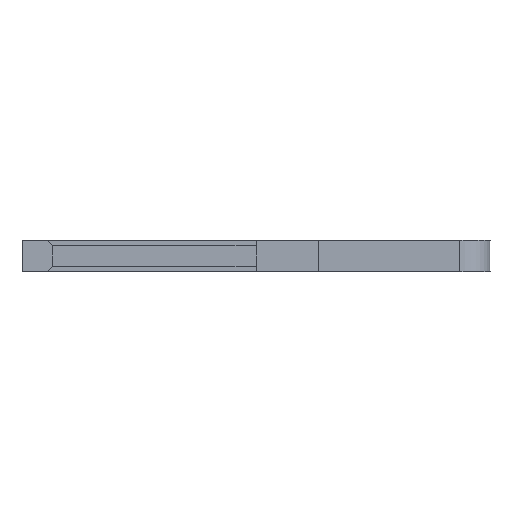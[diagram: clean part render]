
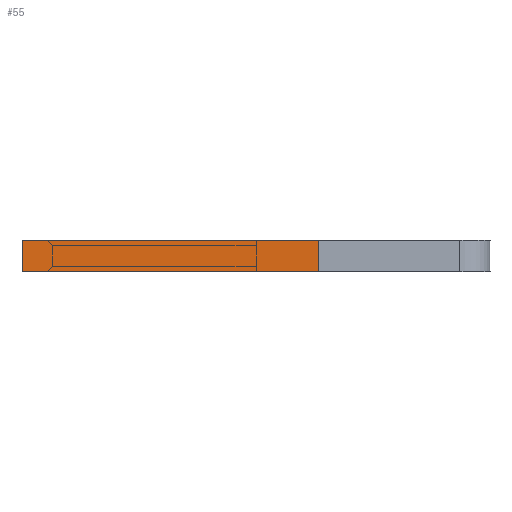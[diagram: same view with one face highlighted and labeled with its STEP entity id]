
A CAD part, left-side view. The second image highlights one B-rep face of the part: STEP entity #55.
In plain terms, the highlighted face is planar.
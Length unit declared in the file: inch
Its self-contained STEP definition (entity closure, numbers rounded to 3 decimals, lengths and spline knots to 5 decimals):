
#55 = ADVANCED_FACE ( 'NONE', ( #3024 ), #1699, .F. ) ;
#84 = ORIENTED_EDGE ( 'NONE', *, *, #358, .F. ) ;
#167 = EDGE_CURVE ( 'NONE', #3244, #1054, #876, .T. ) ;
#208 = CARTESIAN_POINT ( 'NONE',  ( 0.01, -0.04, -0.04 ) ) ;
#341 = CARTESIAN_POINT ( 'NONE',  ( -0.01, 0.15, -0.04 ) ) ;
#358 = EDGE_CURVE ( 'NONE', #1054, #1036, #530, .T. ) ;
#530 = LINE ( 'NONE', #1900, #2147 ) ;
#823 = DIRECTION ( 'NONE',  ( 0., 1., 0. ) ) ;
#876 = LINE ( 'NONE', #1719, #3229 ) ;
#911 = VECTOR ( 'NONE', #939, 39.37008 ) ;
#939 = DIRECTION ( 'NONE',  ( 0., 1., 0. ) ) ;
#1036 = VERTEX_POINT ( 'NONE', #3595 ) ;
#1054 = VERTEX_POINT ( 'NONE', #1191 ) ;
#1191 = CARTESIAN_POINT ( 'NONE',  ( 0.01, 0.15, -0.04 ) ) ;
#1333 = ORIENTED_EDGE ( 'NONE', *, *, #1882, .T. ) ;
#1542 = CARTESIAN_POINT ( 'NONE',  ( 0.01, -0.04, -0.04 ) ) ;
#1699 = PLANE ( 'NONE',  #2333 ) ;
#1719 = CARTESIAN_POINT ( 'NONE',  ( 0.01, 0.15, -0.04 ) ) ;
#1778 = LINE ( 'NONE', #341, #911 ) ;
#1781 = ORIENTED_EDGE ( 'NONE', *, *, #2105, .T. ) ;
#1882 = EDGE_CURVE ( 'NONE', #2648, #1036, #1778, .T. ) ;
#1900 = CARTESIAN_POINT ( 'NONE',  ( 0.01, 0.15, -0.04 ) ) ;
#2011 = DIRECTION ( 'NONE',  ( 1., 0., 0. ) ) ;
#2105 = EDGE_CURVE ( 'NONE', #3244, #2648, #3536, .T. ) ;
#2117 = DIRECTION ( 'NONE',  ( -1., 0., 0. ) ) ;
#2147 = VECTOR ( 'NONE', #2322, 39.37008 ) ;
#2313 = CARTESIAN_POINT ( 'NONE',  ( 0.01, 0.15, -0.04 ) ) ;
#2322 = DIRECTION ( 'NONE',  ( -1., 0., 0. ) ) ;
#2333 = AXIS2_PLACEMENT_3D ( 'NONE', #2313, #3616, #2011 ) ;
#2343 = ORIENTED_EDGE ( 'NONE', *, *, #167, .F. ) ;
#2648 = VERTEX_POINT ( 'NONE', #3107 ) ;
#3024 = FACE_OUTER_BOUND ( 'NONE', #3625, .T. ) ;
#3107 = CARTESIAN_POINT ( 'NONE',  ( -0.01, -0.04, -0.04 ) ) ;
#3229 = VECTOR ( 'NONE', #823, 39.37008 ) ;
#3244 = VERTEX_POINT ( 'NONE', #208 ) ;
#3485 = VECTOR ( 'NONE', #2117, 39.37008 ) ;
#3536 = LINE ( 'NONE', #1542, #3485 ) ;
#3595 = CARTESIAN_POINT ( 'NONE',  ( -0.01, 0.15, -0.04 ) ) ;
#3616 = DIRECTION ( 'NONE',  ( 0., 0., 1. ) ) ;
#3625 = EDGE_LOOP ( 'NONE', ( #1333, #84, #2343, #1781 ) ) ;
